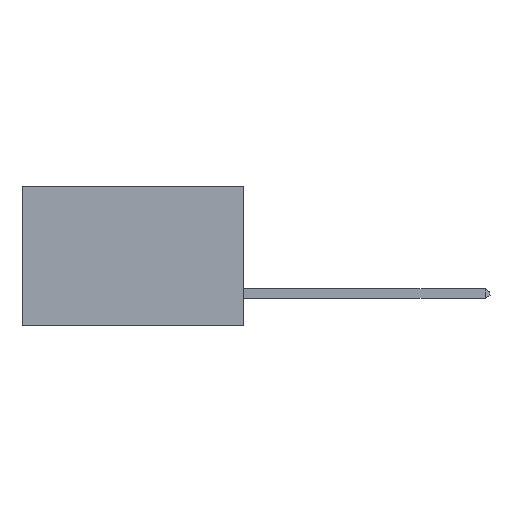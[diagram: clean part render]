
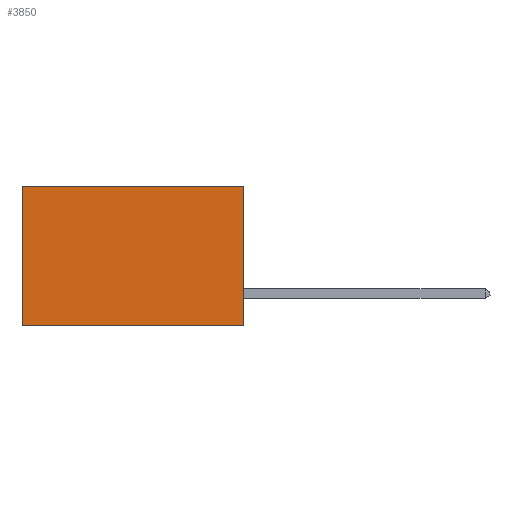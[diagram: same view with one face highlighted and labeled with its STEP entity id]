
A CAD part, left-side view. The second image highlights one B-rep face of the part: STEP entity #3850.
In plain terms, the highlighted planar face has unit normal (-1, 0, 0).
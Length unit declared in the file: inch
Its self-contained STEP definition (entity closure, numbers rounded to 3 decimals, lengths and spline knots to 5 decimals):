
#464 = VECTOR ( 'NONE', #5334, 39.37008 ) ;
#755 = CARTESIAN_POINT ( 'NONE',  ( 0.277, 0., 0. ) ) ;
#799 = LINE ( 'NONE', #10172, #464 ) ;
#1305 = DIRECTION ( 'NONE',  ( 0., 0., -1. ) ) ;
#1828 = DIRECTION ( 'NONE',  ( 0., 1., 0. ) ) ;
#2370 = VERTEX_POINT ( 'NONE', #11508 ) ;
#2396 = CARTESIAN_POINT ( 'NONE',  ( 0.277, 0.59, -0.37 ) ) ;
#2472 = DIRECTION ( 'NONE',  ( 0., 0., -1. ) ) ;
#3850 = ADVANCED_FACE ( 'NONE', ( #7620 ), #9333, .F. ) ;
#4660 = CARTESIAN_POINT ( 'NONE',  ( 0.277, 0.59, 0. ) ) ;
#4726 = ORIENTED_EDGE ( 'NONE', *, *, #5875, .T. ) ;
#4739 = CARTESIAN_POINT ( 'NONE',  ( 0.277, 0.59, -0.37 ) ) ;
#4823 = CARTESIAN_POINT ( 'NONE',  ( 0.277, 0., -0.37 ) ) ;
#4938 = EDGE_CURVE ( 'NONE', #12239, #7155, #10594, .T. ) ;
#5212 = DIRECTION ( 'NONE',  ( 1., 0., 0. ) ) ;
#5334 = DIRECTION ( 'NONE',  ( 0., 1., 0. ) ) ;
#5389 = AXIS2_PLACEMENT_3D ( 'NONE', #9517, #5212, #1305 ) ;
#5805 = DIRECTION ( 'NONE',  ( 0., 0., -1. ) ) ;
#5875 = EDGE_CURVE ( 'NONE', #11285, #12239, #11280, .T. ) ;
#6210 = VECTOR ( 'NONE', #1828, 39.37008 ) ;
#6867 = EDGE_LOOP ( 'NONE', ( #9620, #12749, #12324, #4726 ) ) ;
#7095 = VECTOR ( 'NONE', #5805, 39.37008 ) ;
#7155 = VERTEX_POINT ( 'NONE', #4739 ) ;
#7237 = EDGE_CURVE ( 'NONE', #11285, #2370, #9678, .T. ) ;
#7620 = FACE_OUTER_BOUND ( 'NONE', #6867, .T. ) ;
#7760 = VECTOR ( 'NONE', #2472, 39.37008 ) ;
#9333 = PLANE ( 'NONE',  #5389 ) ;
#9517 = CARTESIAN_POINT ( 'NONE',  ( 0.277, 0., -0.37 ) ) ;
#9620 = ORIENTED_EDGE ( 'NONE', *, *, #4938, .T. ) ;
#9678 = LINE ( 'NONE', #4823, #7095 ) ;
#10172 = CARTESIAN_POINT ( 'NONE',  ( 0.277, 0., -0.37 ) ) ;
#10240 = CARTESIAN_POINT ( 'NONE',  ( 0.277, 0., 0. ) ) ;
#10432 = EDGE_CURVE ( 'NONE', #2370, #7155, #799, .T. ) ;
#10594 = LINE ( 'NONE', #2396, #7760 ) ;
#11280 = LINE ( 'NONE', #755, #6210 ) ;
#11285 = VERTEX_POINT ( 'NONE', #10240 ) ;
#11508 = CARTESIAN_POINT ( 'NONE',  ( 0.277, 0., -0.37 ) ) ;
#12239 = VERTEX_POINT ( 'NONE', #4660 ) ;
#12324 = ORIENTED_EDGE ( 'NONE', *, *, #7237, .F. ) ;
#12749 = ORIENTED_EDGE ( 'NONE', *, *, #10432, .F. ) ;
